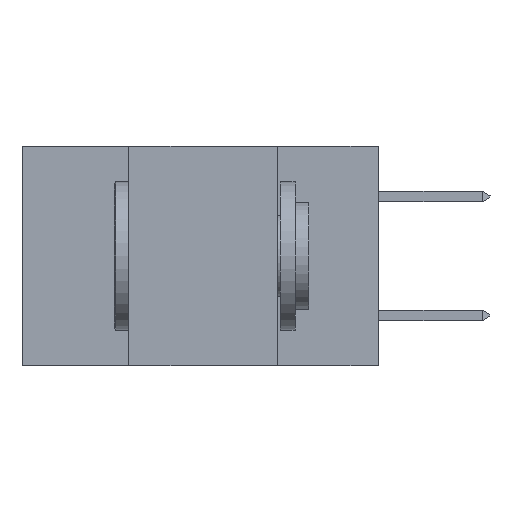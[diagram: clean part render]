
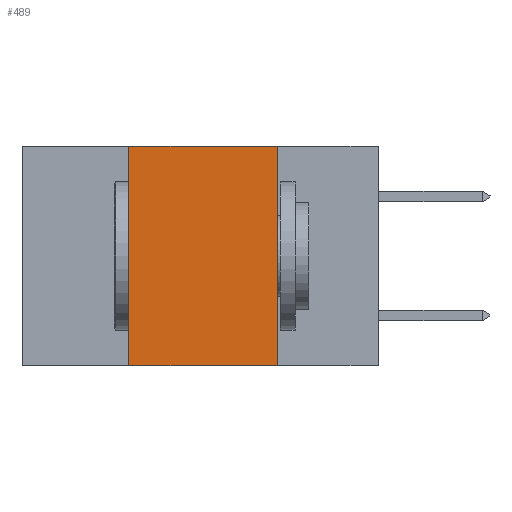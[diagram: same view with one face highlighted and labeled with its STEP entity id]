
A CAD part, left-side view. The second image highlights one B-rep face of the part: STEP entity #489.
In plain terms, the highlighted planar face has unit normal (-1, 0, 0).
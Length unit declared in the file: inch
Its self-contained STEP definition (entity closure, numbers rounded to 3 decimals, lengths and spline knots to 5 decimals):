
#219 = CARTESIAN_POINT ( 'NONE',  ( 0., 0.42, -0.37 ) ) ;
#325 = DIRECTION ( 'NONE',  ( 0., -1., 0. ) ) ;
#489 = ADVANCED_FACE ( 'NONE', ( #8318 ), #11532, .F. ) ;
#1090 = LINE ( 'NONE', #8141, #6861 ) ;
#1957 = VERTEX_POINT ( 'NONE', #3181 ) ;
#2519 = EDGE_CURVE ( 'NONE', #4260, #3799, #1090, .T. ) ;
#2605 = ORIENTED_EDGE ( 'NONE', *, *, #10986, .F. ) ;
#3181 = CARTESIAN_POINT ( 'NONE',  ( 0., 0.42, 0. ) ) ;
#3799 = VERTEX_POINT ( 'NONE', #4311 ) ;
#4260 = VERTEX_POINT ( 'NONE', #7587 ) ;
#4311 = CARTESIAN_POINT ( 'NONE',  ( 0., 0.17, -0.37 ) ) ;
#4376 = ORIENTED_EDGE ( 'NONE', *, *, #9702, .F. ) ;
#4610 = DIRECTION ( 'NONE',  ( 0., 0., -1. ) ) ;
#4897 = LINE ( 'NONE', #11775, #7754 ) ;
#5205 = VERTEX_POINT ( 'NONE', #13354 ) ;
#5975 = CARTESIAN_POINT ( 'NONE',  ( 0., 0.6, 0. ) ) ;
#6275 = VECTOR ( 'NONE', #9525, 39.37008 ) ;
#6861 = VECTOR ( 'NONE', #4610, 39.37008 ) ;
#7587 = CARTESIAN_POINT ( 'NONE',  ( 0., 0.17, 0. ) ) ;
#7754 = VECTOR ( 'NONE', #325, 39.37008 ) ;
#8141 = CARTESIAN_POINT ( 'NONE',  ( 0., 0.17, -0.37 ) ) ;
#8318 = FACE_OUTER_BOUND ( 'NONE', #8373, .T. ) ;
#8373 = EDGE_LOOP ( 'NONE', ( #8621, #2605, #4376, #11866 ) ) ;
#8621 = ORIENTED_EDGE ( 'NONE', *, *, #2519, .F. ) ;
#9525 = DIRECTION ( 'NONE',  ( 0., 0., 1. ) ) ;
#9630 = LINE ( 'NONE', #13061, #11289 ) ;
#9702 = EDGE_CURVE ( 'NONE', #5205, #1957, #10697, .T. ) ;
#9707 = DIRECTION ( 'NONE',  ( 0., -1., 0. ) ) ;
#10697 = LINE ( 'NONE', #219, #6275 ) ;
#10986 = EDGE_CURVE ( 'NONE', #1957, #4260, #9630, .T. ) ;
#11289 = VECTOR ( 'NONE', #9707, 39.37008 ) ;
#11532 = PLANE ( 'NONE',  #14845 ) ;
#11775 = CARTESIAN_POINT ( 'NONE',  ( 0., 0.6, -0.37 ) ) ;
#11866 = ORIENTED_EDGE ( 'NONE', *, *, #13523, .T. ) ;
#12659 = DIRECTION ( 'NONE',  ( 0., 0., -1. ) ) ;
#13061 = CARTESIAN_POINT ( 'NONE',  ( 0., 0.6, 0. ) ) ;
#13354 = CARTESIAN_POINT ( 'NONE',  ( 0., 0.42, -0.37 ) ) ;
#13523 = EDGE_CURVE ( 'NONE', #5205, #3799, #4897, .T. ) ;
#13817 = DIRECTION ( 'NONE',  ( 1., 0., 0. ) ) ;
#14845 = AXIS2_PLACEMENT_3D ( 'NONE', #5975, #13817, #12659 ) ;
